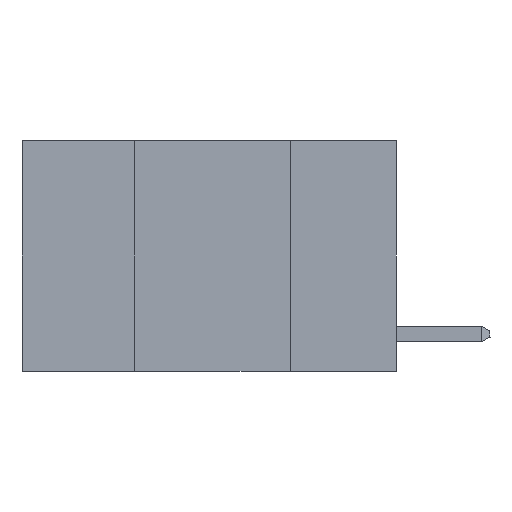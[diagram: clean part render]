
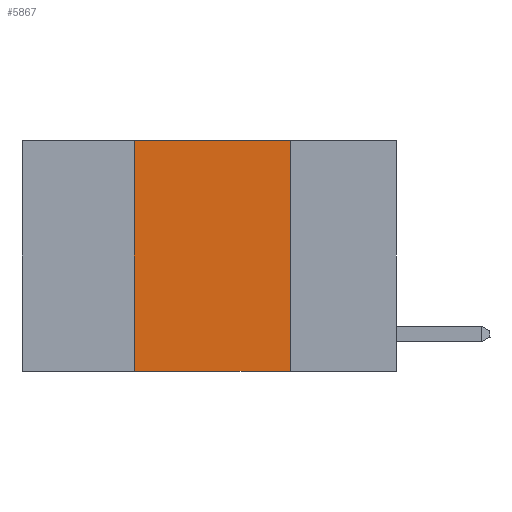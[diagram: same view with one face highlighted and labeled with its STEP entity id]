
A CAD part, left-side view. The second image highlights one B-rep face of the part: STEP entity #5867.
In plain terms, the highlighted planar face has unit normal (-1, 0, 0).
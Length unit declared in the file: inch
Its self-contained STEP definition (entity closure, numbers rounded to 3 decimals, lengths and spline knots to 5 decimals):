
#205 = AXIS2_PLACEMENT_3D ( 'NONE', #10568, #7135, #15035 ) ;
#1004 = VERTEX_POINT ( 'NONE', #3469 ) ;
#1977 = ORIENTED_EDGE ( 'NONE', *, *, #7132, .T. ) ;
#2148 = VECTOR ( 'NONE', #8666, 39.37008 ) ;
#2161 = CARTESIAN_POINT ( 'NONE',  ( 0., 0.42, 0. ) ) ;
#2467 = EDGE_CURVE ( 'NONE', #4378, #4388, #6679, .T. ) ;
#3112 = ORIENTED_EDGE ( 'NONE', *, *, #8043, .F. ) ;
#3469 = CARTESIAN_POINT ( 'NONE',  ( 0., 0.42, -0.37 ) ) ;
#3870 = FACE_OUTER_BOUND ( 'NONE', #8660, .T. ) ;
#4378 = VERTEX_POINT ( 'NONE', #12364 ) ;
#4388 = VERTEX_POINT ( 'NONE', #10209 ) ;
#4725 = PLANE ( 'NONE',  #205 ) ;
#5515 = CARTESIAN_POINT ( 'NONE',  ( 0., 0.17, 0. ) ) ;
#5860 = VECTOR ( 'NONE', #13769, 39.37008 ) ;
#5867 = ADVANCED_FACE ( 'NONE', ( #3870 ), #4725, .F. ) ;
#5902 = ORIENTED_EDGE ( 'NONE', *, *, #8802, .F. ) ;
#5937 = VECTOR ( 'NONE', #14948, 39.37008 ) ;
#6231 = LINE ( 'NONE', #2161, #5860 ) ;
#6288 = CARTESIAN_POINT ( 'NONE',  ( 0., 0.17, -0.37 ) ) ;
#6679 = LINE ( 'NONE', #10579, #5937 ) ;
#6726 = DIRECTION ( 'NONE',  ( 0., 0., -1. ) ) ;
#7132 = EDGE_CURVE ( 'NONE', #1004, #8453, #11476, .T. ) ;
#7135 = DIRECTION ( 'NONE',  ( 1., 0., 0. ) ) ;
#7946 = VECTOR ( 'NONE', #6726, 39.37008 ) ;
#8043 = EDGE_CURVE ( 'NONE', #4388, #8453, #13933, .T. ) ;
#8453 = VERTEX_POINT ( 'NONE', #6288 ) ;
#8660 = EDGE_LOOP ( 'NONE', ( #3112, #14296, #5902, #1977 ) ) ;
#8666 = DIRECTION ( 'NONE',  ( 0., -1., 0. ) ) ;
#8802 = EDGE_CURVE ( 'NONE', #1004, #4378, #6231, .T. ) ;
#9821 = CARTESIAN_POINT ( 'NONE',  ( 0., 0.6, -0.37 ) ) ;
#10209 = CARTESIAN_POINT ( 'NONE',  ( 0., 0.17, 0. ) ) ;
#10568 = CARTESIAN_POINT ( 'NONE',  ( 0., 0.6, 0. ) ) ;
#10579 = CARTESIAN_POINT ( 'NONE',  ( 0., 0.6, 0. ) ) ;
#11476 = LINE ( 'NONE', #9821, #2148 ) ;
#12364 = CARTESIAN_POINT ( 'NONE',  ( 0., 0.42, 0. ) ) ;
#13769 = DIRECTION ( 'NONE',  ( 0., 0., 1. ) ) ;
#13933 = LINE ( 'NONE', #5515, #7946 ) ;
#14296 = ORIENTED_EDGE ( 'NONE', *, *, #2467, .F. ) ;
#14948 = DIRECTION ( 'NONE',  ( 0., -1., 0. ) ) ;
#15035 = DIRECTION ( 'NONE',  ( 0., 0., -1. ) ) ;
